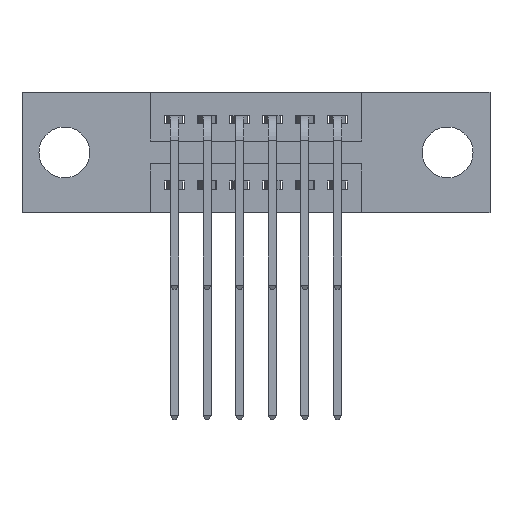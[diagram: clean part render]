
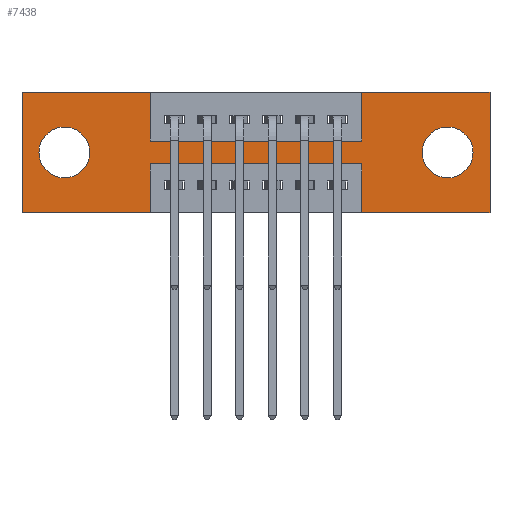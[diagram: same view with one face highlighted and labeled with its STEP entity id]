
A CAD part, front view. The second image highlights one B-rep face of the part: STEP entity #7438.
In plain terms, the highlighted planar face has unit normal (0, -1, 0).
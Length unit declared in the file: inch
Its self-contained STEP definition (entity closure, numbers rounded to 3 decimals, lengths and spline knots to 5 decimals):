
#58 = EDGE_CURVE ( 'NONE', #6432, #7984, #8761, .T. ) ;
#72 = DIRECTION ( 'NONE',  ( 0., 0., 1. ) ) ;
#208 = DIRECTION ( 'NONE',  ( -1., 0., 0. ) ) ;
#234 = ORIENTED_EDGE ( 'NONE', *, *, #9894, .F. ) ;
#328 = CARTESIAN_POINT ( 'NONE',  ( 0.3925, 0., 0. ) ) ;
#417 = CARTESIAN_POINT ( 'NONE',  ( 0.3925, 0., -0.37 ) ) ;
#694 = CARTESIAN_POINT ( 'NONE',  ( 0., 0., -0.37 ) ) ;
#744 = CARTESIAN_POINT ( 'NONE',  ( 1.305, 0., -0.263 ) ) ;
#757 = DIRECTION ( 'NONE',  ( 0., 0., 1. ) ) ;
#760 = EDGE_CURVE ( 'NONE', #4789, #6448, #9180, .T. ) ;
#798 = LINE ( 'NONE', #9040, #2676 ) ;
#865 = LINE ( 'NONE', #4443, #7859 ) ;
#873 = DIRECTION ( 'NONE',  ( -1., 0., 0. ) ) ;
#1120 = EDGE_CURVE ( 'NONE', #10124, #5079, #1746, .T. ) ;
#1566 = EDGE_CURVE ( 'NONE', #7091, #4009, #865, .T. ) ;
#1604 = ORIENTED_EDGE ( 'NONE', *, *, #10332, .T. ) ;
#1699 = EDGE_CURVE ( 'NONE', #3097, #9783, #9277, .T. ) ;
#1746 = LINE ( 'NONE', #8949, #2272 ) ;
#2004 = DIRECTION ( 'NONE',  ( 0., 1., 0. ) ) ;
#2087 = DIRECTION ( 'NONE',  ( 0., 0., -1. ) ) ;
#2092 = CIRCLE ( 'NONE', #6252, 0.078 ) ;
#2131 = VECTOR ( 'NONE', #9759, 39.37008 ) ;
#2157 = ORIENTED_EDGE ( 'NONE', *, *, #5027, .F. ) ;
#2272 = VECTOR ( 'NONE', #873, 39.37008 ) ;
#2290 = ORIENTED_EDGE ( 'NONE', *, *, #760, .F. ) ;
#2363 = DIRECTION ( 'NONE',  ( 0., 0., -1. ) ) ;
#2365 = FACE_OUTER_BOUND ( 'NONE', #3206, .T. ) ;
#2674 = EDGE_CURVE ( 'NONE', #9669, #5003, #4172, .T. ) ;
#2676 = VECTOR ( 'NONE', #11636, 39.37008 ) ;
#2681 = AXIS2_PLACEMENT_3D ( 'NONE', #6976, #7087, #2363 ) ;
#2711 = VERTEX_POINT ( 'NONE', #9656 ) ;
#2879 = AXIS2_PLACEMENT_3D ( 'NONE', #7080, #6195, #72 ) ;
#2899 = DIRECTION ( 'NONE',  ( 1., 0., 0. ) ) ;
#3029 = VERTEX_POINT ( 'NONE', #744 ) ;
#3081 = ORIENTED_EDGE ( 'NONE', *, *, #9461, .F. ) ;
#3097 = VERTEX_POINT ( 'NONE', #6811 ) ;
#3134 = CARTESIAN_POINT ( 'NONE',  ( 0., 0., 0. ) ) ;
#3193 = CARTESIAN_POINT ( 'NONE',  ( 1.435, 0., -0.37 ) ) ;
#3201 = ORIENTED_EDGE ( 'NONE', *, *, #7232, .F. ) ;
#3206 = EDGE_LOOP ( 'NONE', ( #8063, #4778, #10775, #2290, #2157, #3081, #11132, #234, #10866, #3201, #9301, #9444 ) ) ;
#3274 = EDGE_CURVE ( 'NONE', #5079, #4961, #798, .T. ) ;
#3305 = CARTESIAN_POINT ( 'NONE',  ( 1.305, 0., -0.185 ) ) ;
#3499 = LINE ( 'NONE', #11528, #2131 ) ;
#3732 = DIRECTION ( 'NONE',  ( 0., 0., 1. ) ) ;
#3909 = DIRECTION ( 'NONE',  ( 0., 0., -1. ) ) ;
#3986 = CARTESIAN_POINT ( 'NONE',  ( 1.435, 0., 0. ) ) ;
#4009 = VERTEX_POINT ( 'NONE', #9012 ) ;
#4172 = LINE ( 'NONE', #10658, #7668 ) ;
#4198 = DIRECTION ( 'NONE',  ( 1., 0., 0. ) ) ;
#4342 = AXIS2_PLACEMENT_3D ( 'NONE', #11463, #6980, #6092 ) ;
#4443 = CARTESIAN_POINT ( 'NONE',  ( 0., 0., 0. ) ) ;
#4444 = EDGE_CURVE ( 'NONE', #4961, #7091, #4999, .T. ) ;
#4548 = EDGE_LOOP ( 'NONE', ( #11535, #1604 ) ) ;
#4653 = CARTESIAN_POINT ( 'NONE',  ( 1.0425, 0., -0.22 ) ) ;
#4725 = CARTESIAN_POINT ( 'NONE',  ( 1.0425, 0., -0.15 ) ) ;
#4778 = ORIENTED_EDGE ( 'NONE', *, *, #1120, .F. ) ;
#4789 = VERTEX_POINT ( 'NONE', #3193 ) ;
#4877 = VECTOR ( 'NONE', #208, 39.37008 ) ;
#4904 = LINE ( 'NONE', #3134, #9418 ) ;
#4961 = VERTEX_POINT ( 'NONE', #417 ) ;
#4999 = LINE ( 'NONE', #10934, #4877 ) ;
#5003 = VERTEX_POINT ( 'NONE', #7532 ) ;
#5011 = DIRECTION ( 'NONE',  ( 0., 1., 0. ) ) ;
#5027 = EDGE_CURVE ( 'NONE', #2711, #4789, #10246, .T. ) ;
#5079 = VERTEX_POINT ( 'NONE', #9295 ) ;
#5329 = LINE ( 'NONE', #10650, #11357 ) ;
#5472 = CARTESIAN_POINT ( 'NONE',  ( 0., 0., -0.37 ) ) ;
#5691 = AXIS2_PLACEMENT_3D ( 'NONE', #9098, #2004, #3732 ) ;
#5692 = DIRECTION ( 'NONE',  ( -1., 0., 0. ) ) ;
#5697 = CARTESIAN_POINT ( 'NONE',  ( 0.13, 0., -0.107 ) ) ;
#5731 = CARTESIAN_POINT ( 'NONE',  ( 0.3925, 0., -0.15 ) ) ;
#5815 = CARTESIAN_POINT ( 'NONE',  ( 0.13, 0., -0.263 ) ) ;
#5886 = CARTESIAN_POINT ( 'NONE',  ( 1.0425, 0., -0.37 ) ) ;
#6092 = DIRECTION ( 'NONE',  ( 0., 0., -1. ) ) ;
#6195 = DIRECTION ( 'NONE',  ( 0., 1., 0. ) ) ;
#6252 = AXIS2_PLACEMENT_3D ( 'NONE', #3305, #5011, #8609 ) ;
#6432 = VERTEX_POINT ( 'NONE', #5697 ) ;
#6448 = VERTEX_POINT ( 'NONE', #5886 ) ;
#6811 = CARTESIAN_POINT ( 'NONE',  ( 0.3925, 0., 0. ) ) ;
#6976 = CARTESIAN_POINT ( 'NONE',  ( 1.305, 0., -0.185 ) ) ;
#6980 = DIRECTION ( 'NONE',  ( 0., -1., 0. ) ) ;
#7080 = CARTESIAN_POINT ( 'NONE',  ( 0.13, 0., -0.185 ) ) ;
#7087 = DIRECTION ( 'NONE',  ( 0., 1., 0. ) ) ;
#7091 = VERTEX_POINT ( 'NONE', #694 ) ;
#7140 = VERTEX_POINT ( 'NONE', #8100 ) ;
#7232 = EDGE_CURVE ( 'NONE', #4009, #3097, #4904, .T. ) ;
#7381 = ORIENTED_EDGE ( 'NONE', *, *, #58, .T. ) ;
#7437 = ORIENTED_EDGE ( 'NONE', *, *, #10852, .T. ) ;
#7438 = ADVANCED_FACE ( 'NONE', ( #7863, #10463, #2365 ), #7804, .T. ) ;
#7532 = CARTESIAN_POINT ( 'NONE',  ( 1.0425, 0., 0. ) ) ;
#7668 = VECTOR ( 'NONE', #757, 39.37008 ) ;
#7735 = VECTOR ( 'NONE', #5692, 39.37008 ) ;
#7804 = PLANE ( 'NONE',  #4342 ) ;
#7859 = VECTOR ( 'NONE', #8051, 39.37008 ) ;
#7863 = FACE_BOUND ( 'NONE', #4548, .T. ) ;
#7984 = VERTEX_POINT ( 'NONE', #5815 ) ;
#7990 = DIRECTION ( 'NONE',  ( 0., 0., 1. ) ) ;
#8051 = DIRECTION ( 'NONE',  ( 0., 0., 1. ) ) ;
#8063 = ORIENTED_EDGE ( 'NONE', *, *, #3274, .F. ) ;
#8100 = CARTESIAN_POINT ( 'NONE',  ( 1.305, 0., -0.107 ) ) ;
#8160 = CIRCLE ( 'NONE', #2681, 0.078 ) ;
#8180 = VECTOR ( 'NONE', #4198, 39.37008 ) ;
#8438 = VECTOR ( 'NONE', #2087, 39.37008 ) ;
#8609 = DIRECTION ( 'NONE',  ( 0., 0., -1. ) ) ;
#8742 = CARTESIAN_POINT ( 'NONE',  ( 0.3925, 0., -0.15 ) ) ;
#8761 = CIRCLE ( 'NONE', #2879, 0.078 ) ;
#8949 = CARTESIAN_POINT ( 'NONE',  ( 0.3925, 0., -0.22 ) ) ;
#9012 = CARTESIAN_POINT ( 'NONE',  ( 0., 0., 0. ) ) ;
#9040 = CARTESIAN_POINT ( 'NONE',  ( 0.3925, 0., -0.37 ) ) ;
#9098 = CARTESIAN_POINT ( 'NONE',  ( 0.13, 0., -0.185 ) ) ;
#9180 = LINE ( 'NONE', #5472, #7735 ) ;
#9277 = LINE ( 'NONE', #328, #11247 ) ;
#9295 = CARTESIAN_POINT ( 'NONE',  ( 0.3925, 0., -0.22 ) ) ;
#9301 = ORIENTED_EDGE ( 'NONE', *, *, #1566, .F. ) ;
#9418 = VECTOR ( 'NONE', #2899, 39.37008 ) ;
#9444 = ORIENTED_EDGE ( 'NONE', *, *, #4444, .F. ) ;
#9461 = EDGE_CURVE ( 'NONE', #5003, #2711, #3499, .T. ) ;
#9628 = LINE ( 'NONE', #8742, #8180 ) ;
#9656 = CARTESIAN_POINT ( 'NONE',  ( 1.435, 0., 0. ) ) ;
#9669 = VERTEX_POINT ( 'NONE', #4725 ) ;
#9699 = EDGE_LOOP ( 'NONE', ( #7381, #7437 ) ) ;
#9759 = DIRECTION ( 'NONE',  ( 1., 0., 0. ) ) ;
#9783 = VERTEX_POINT ( 'NONE', #5731 ) ;
#9894 = EDGE_CURVE ( 'NONE', #9783, #9669, #9628, .T. ) ;
#10124 = VERTEX_POINT ( 'NONE', #4653 ) ;
#10217 = CIRCLE ( 'NONE', #5691, 0.078 ) ;
#10246 = LINE ( 'NONE', #3986, #8438 ) ;
#10332 = EDGE_CURVE ( 'NONE', #3029, #7140, #2092, .T. ) ;
#10463 = FACE_BOUND ( 'NONE', #9699, .T. ) ;
#10650 = CARTESIAN_POINT ( 'NONE',  ( 1.0425, 0., -0.37 ) ) ;
#10658 = CARTESIAN_POINT ( 'NONE',  ( 1.0425, 0., 0. ) ) ;
#10694 = EDGE_CURVE ( 'NONE', #6448, #10124, #5329, .T. ) ;
#10775 = ORIENTED_EDGE ( 'NONE', *, *, #10694, .F. ) ;
#10852 = EDGE_CURVE ( 'NONE', #7984, #6432, #10217, .T. ) ;
#10866 = ORIENTED_EDGE ( 'NONE', *, *, #1699, .F. ) ;
#10934 = CARTESIAN_POINT ( 'NONE',  ( 0., 0., -0.37 ) ) ;
#11123 = EDGE_CURVE ( 'NONE', #7140, #3029, #8160, .T. ) ;
#11132 = ORIENTED_EDGE ( 'NONE', *, *, #2674, .F. ) ;
#11247 = VECTOR ( 'NONE', #3909, 39.37008 ) ;
#11357 = VECTOR ( 'NONE', #7990, 39.37008 ) ;
#11463 = CARTESIAN_POINT ( 'NONE',  ( 0., 0., -0.37 ) ) ;
#11528 = CARTESIAN_POINT ( 'NONE',  ( 0., 0., 0. ) ) ;
#11535 = ORIENTED_EDGE ( 'NONE', *, *, #11123, .T. ) ;
#11636 = DIRECTION ( 'NONE',  ( 0., 0., -1. ) ) ;
